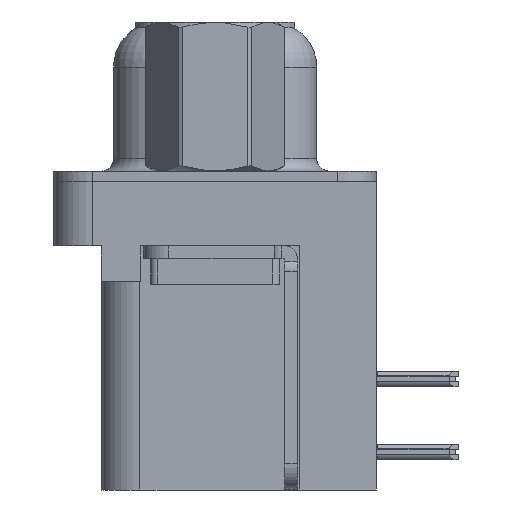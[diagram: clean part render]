
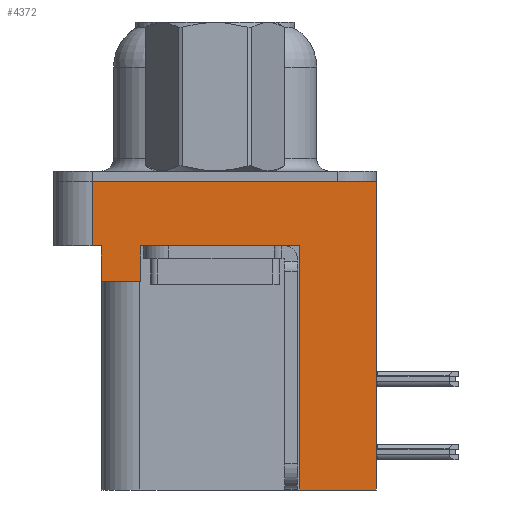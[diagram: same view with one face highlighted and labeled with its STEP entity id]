
A CAD part, left-side view. The second image highlights one B-rep face of the part: STEP entity #4372.
In plain terms, the highlighted planar face has unit normal (-1, 0, 0).
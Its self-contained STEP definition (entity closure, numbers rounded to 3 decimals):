
#662 = CARTESIAN_POINT ( 'NONE',  ( -2.91, -6.275, -2.5 ) ) ;
#1059 = EDGE_CURVE ( 'NONE', #31802, #3843, #27706, .T. ) ;
#1153 = ORIENTED_EDGE ( 'NONE', *, *, #5818, .F. ) ;
#1623 = ORIENTED_EDGE ( 'NONE', *, *, #4395, .F. ) ;
#2150 = EDGE_CURVE ( 'NONE', #3843, #2361, #4073, .T. ) ;
#2361 = VERTEX_POINT ( 'NONE', #15169 ) ;
#3843 = VERTEX_POINT ( 'NONE', #6365 ) ;
#4014 = EDGE_CURVE ( 'NONE', #31802, #19384, #39767, .T. ) ;
#4073 = LINE ( 'NONE', #17004, #33938 ) ;
#4372 = ADVANCED_FACE ( 'NONE', ( #16752 ), #27422, .T. ) ;
#4395 = EDGE_CURVE ( 'NONE', #33767, #28088, #7405, .T. ) ;
#4463 = DIRECTION ( 'NONE',  ( 0., 0., 1. ) ) ;
#5610 = DIRECTION ( 'NONE',  ( 0., 0., 1. ) ) ;
#5616 = VERTEX_POINT ( 'NONE', #19641 ) ;
#5752 = CARTESIAN_POINT ( 'NONE',  ( -2.91, -3.295, -12. ) ) ;
#5818 = EDGE_CURVE ( 'NONE', #28088, #11109, #25922, .T. ) ;
#6114 = CARTESIAN_POINT ( 'NONE',  ( -2.91, -3.295, -12. ) ) ;
#6365 = CARTESIAN_POINT ( 'NONE',  ( -2.91, 4.425, -3.9 ) ) ;
#6862 = DIRECTION ( 'NONE',  ( 0., 0., 1. ) ) ;
#7138 = VECTOR ( 'NONE', #6862, 1000. ) ;
#7405 = LINE ( 'NONE', #5752, #8417 ) ;
#8088 = VECTOR ( 'NONE', #19819, 1000. ) ;
#8296 = ORIENTED_EDGE ( 'NONE', *, *, #37448, .F. ) ;
#8417 = VECTOR ( 'NONE', #8813, 1000. ) ;
#8539 = CARTESIAN_POINT ( 'NONE',  ( -2.91, -6.275, -2.5 ) ) ;
#8813 = DIRECTION ( 'NONE',  ( 0., 1., 0. ) ) ;
#9285 = CARTESIAN_POINT ( 'NONE',  ( -2.91, 2.895, -2.5 ) ) ;
#9296 = VECTOR ( 'NONE', #23332, 1000. ) ;
#9826 = DIRECTION ( 'NONE',  ( 0., -1., 0. ) ) ;
#10908 = VECTOR ( 'NONE', #19407, 1000. ) ;
#11109 = VERTEX_POINT ( 'NONE', #40511 ) ;
#12243 = DIRECTION ( 'NONE',  ( -1., 0., 0. ) ) ;
#13077 = CARTESIAN_POINT ( 'NONE',  ( -2.91, 2.895, -3.9 ) ) ;
#13420 = DIRECTION ( 'NONE',  ( 0., -1., 0. ) ) ;
#13977 = ORIENTED_EDGE ( 'NONE', *, *, #1059, .F. ) ;
#15169 = CARTESIAN_POINT ( 'NONE',  ( -2.91, 4.425, -2.5 ) ) ;
#15475 = LINE ( 'NONE', #19388, #7138 ) ;
#15549 = ORIENTED_EDGE ( 'NONE', *, *, #4014, .T. ) ;
#15551 = ORIENTED_EDGE ( 'NONE', *, *, #2150, .F. ) ;
#15686 = CARTESIAN_POINT ( 'NONE',  ( -2.91, -6.275, -2.5 ) ) ;
#15779 = VERTEX_POINT ( 'NONE', #30825 ) ;
#16752 = FACE_OUTER_BOUND ( 'NONE', #40083, .T. ) ;
#17004 = CARTESIAN_POINT ( 'NONE',  ( -2.91, 4.425, -3.9 ) ) ;
#17012 = CARTESIAN_POINT ( 'NONE',  ( -2.91, 2.895, -3.9 ) ) ;
#19384 = VERTEX_POINT ( 'NONE', #9285 ) ;
#19388 = CARTESIAN_POINT ( 'NONE',  ( -2.91, -6.275, -2.5 ) ) ;
#19407 = DIRECTION ( 'NONE',  ( 0., 0., 1. ) ) ;
#19453 = EDGE_CURVE ( 'NONE', #19384, #11109, #31941, .T. ) ;
#19641 = CARTESIAN_POINT ( 'NONE',  ( -2.91, 4.775, 0. ) ) ;
#19819 = DIRECTION ( 'NONE',  ( 0., 0., 1. ) ) ;
#20276 = DIRECTION ( 'NONE',  ( 0., 1., 0. ) ) ;
#22828 = EDGE_CURVE ( 'NONE', #15779, #2361, #33978, .T. ) ;
#22863 = VERTEX_POINT ( 'NONE', #37867 ) ;
#23332 = DIRECTION ( 'NONE',  ( 0., 0., 1. ) ) ;
#23715 = VECTOR ( 'NONE', #27737, 1000. ) ;
#24927 = ORIENTED_EDGE ( 'NONE', *, *, #22828, .T. ) ;
#25922 = LINE ( 'NONE', #26480, #9296 ) ;
#26173 = VECTOR ( 'NONE', #13420, 1000. ) ;
#26480 = CARTESIAN_POINT ( 'NONE',  ( -2.91, -3.295, -12. ) ) ;
#26746 = CARTESIAN_POINT ( 'NONE',  ( -2.91, -6.275, -12. ) ) ;
#26760 = VECTOR ( 'NONE', #9826, 1000. ) ;
#27422 = PLANE ( 'NONE',  #29926 ) ;
#27706 = LINE ( 'NONE', #32654, #34482 ) ;
#27737 = DIRECTION ( 'NONE',  ( 0., -1., 0. ) ) ;
#28088 = VERTEX_POINT ( 'NONE', #6114 ) ;
#28408 = CARTESIAN_POINT ( 'NONE',  ( -2.91, -6.275, 0. ) ) ;
#28517 = CARTESIAN_POINT ( 'NONE',  ( -2.91, 4.775, -2.5 ) ) ;
#29926 = AXIS2_PLACEMENT_3D ( 'NONE', #8539, #12243, #5610 ) ;
#30139 = ORIENTED_EDGE ( 'NONE', *, *, #37902, .T. ) ;
#30825 = CARTESIAN_POINT ( 'NONE',  ( -2.91, 4.775, -2.5 ) ) ;
#31526 = ORIENTED_EDGE ( 'NONE', *, *, #33600, .F. ) ;
#31802 = VERTEX_POINT ( 'NONE', #17012 ) ;
#31941 = LINE ( 'NONE', #15686, #23715 ) ;
#32654 = CARTESIAN_POINT ( 'NONE',  ( -2.91, 4.425, -3.9 ) ) ;
#33600 = EDGE_CURVE ( 'NONE', #5616, #22863, #36472, .T. ) ;
#33767 = VERTEX_POINT ( 'NONE', #26746 ) ;
#33938 = VECTOR ( 'NONE', #4463, 1000. ) ;
#33978 = LINE ( 'NONE', #662, #26173 ) ;
#34412 = LINE ( 'NONE', #28517, #8088 ) ;
#34482 = VECTOR ( 'NONE', #20276, 1000. ) ;
#36472 = LINE ( 'NONE', #28408, #26760 ) ;
#37448 = EDGE_CURVE ( 'NONE', #15779, #5616, #34412, .T. ) ;
#37867 = CARTESIAN_POINT ( 'NONE',  ( -2.91, -6.275, 0. ) ) ;
#37902 = EDGE_CURVE ( 'NONE', #33767, #22863, #15475, .T. ) ;
#39767 = LINE ( 'NONE', #13077, #10908 ) ;
#40083 = EDGE_LOOP ( 'NONE', ( #31526, #8296, #24927, #15551, #13977, #15549, #40534, #1153, #1623, #30139 ) ) ;
#40511 = CARTESIAN_POINT ( 'NONE',  ( -2.91, -3.295, -2.5 ) ) ;
#40534 = ORIENTED_EDGE ( 'NONE', *, *, #19453, .T. ) ;
